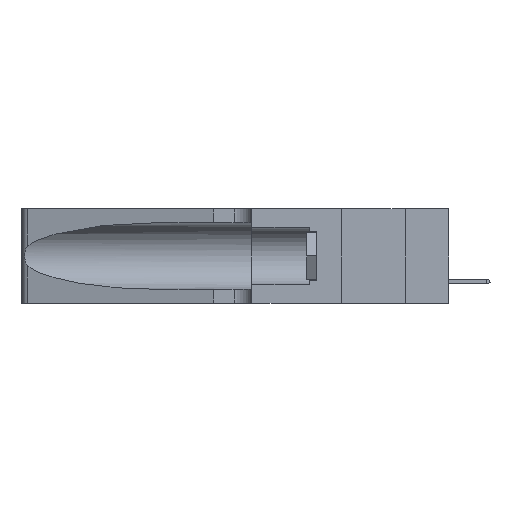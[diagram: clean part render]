
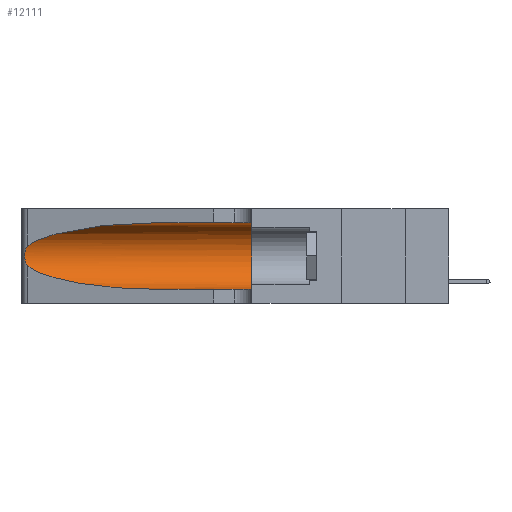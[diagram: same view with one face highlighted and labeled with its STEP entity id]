
A CAD part, left-side view. The second image highlights one B-rep face of the part: STEP entity #12111.
In plain terms, the highlighted cylindrical face has radius 3.308 mm (diameter 6.617 mm), a partial arc.
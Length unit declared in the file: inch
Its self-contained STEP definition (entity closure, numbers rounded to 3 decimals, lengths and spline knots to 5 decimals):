
#416 = CIRCLE ( 'NONE', #11022, 0.13025 ) ;
#434 = CARTESIAN_POINT ( 'NONE',  ( 0.1305, 0.72297, 0.31525 ) ) ;
#457 = DIRECTION ( 'NONE',  ( 0., 0., -1. ) ) ;
#665 = DIRECTION ( 'NONE',  ( 0., -1., 0. ) ) ;
#813 = CARTESIAN_POINT ( 'NONE',  ( 0.1305, 1.61858, 0.05475 ) ) ;
#1003 = EDGE_CURVE ( 'NONE', #6427, #7601, #4981, .T. ) ;
#2131 = CARTESIAN_POINT ( 'NONE',  ( 0.1305, 0.35, 0.185 ) ) ;
#2793 = LINE ( 'NONE', #813, #10927 ) ;
#2992 = EDGE_LOOP ( 'NONE', ( #15662, #5739, #11765, #10380, #9431, #17140 ) ) ;
#3271 = B_SPLINE_CURVE_WITH_KNOTS ( 'NONE', 3,
 ( #14255, #17311, #11623, #3911, #15981, #14503, #13169, #16174, #19158, #14706, #19229, #11430, #14574, #17772 ),
 .UNSPECIFIED., .F., .F.,
 ( 4, 2, 2, 2, 2, 2, 4 ),
 ( 0., 0.00027, 0.00053, 0.00107, 0.0016, 0.00187, 0.00214 ),
 .UNSPECIFIED. ) ;
#3377 = EDGE_CURVE ( 'NONE', #10910, #6811, #11810, .T. ) ;
#3838 = DIRECTION ( 'NONE',  ( 0., -1., 0. ) ) ;
#3911 = CARTESIAN_POINT ( 'NONE',  ( 0.25787, 1.23484, 0.2124 ) ) ;
#4242 = CARTESIAN_POINT ( 'NONE',  ( 0.1305, 1.61858, 0.185 ) ) ;
#4283 = EDGE_CURVE ( 'NONE', #7601, #10910, #3271, .T. ) ;
#4562 = CARTESIAN_POINT ( 'NONE',  ( 0.1305, 0.72297, 0.05475 ) ) ;
#4981 =( BOUNDED_CURVE ( )  B_SPLINE_CURVE ( 3, ( #434, #18572, #14188, #14113 ),
 .UNSPECIFIED., .F., .T. ) 
 B_SPLINE_CURVE_WITH_KNOTS ( ( 4, 4 ),
 ( 1.5708, 2.84003 ),
 .UNSPECIFIED. ) 
 CURVE ( )  GEOMETRIC_REPRESENTATION_ITEM ( )  RATIONAL_B_SPLINE_CURVE ( ( 1., 0.87, 0.87, 1. ) ) 
 REPRESENTATION_ITEM ( '' )  );
#5599 = CARTESIAN_POINT ( 'NONE',  ( 0.1305, 0.35, 0.05475 ) ) ;
#5739 = ORIENTED_EDGE ( 'NONE', *, *, #4283, .T. ) ;
#5906 = VERTEX_POINT ( 'NONE', #5599 ) ;
#6427 = VERTEX_POINT ( 'NONE', #9288 ) ;
#6769 = CYLINDRICAL_SURFACE ( 'NONE', #19738, 0.13025 ) ;
#6794 = EDGE_CURVE ( 'NONE', #6427, #15471, #12425, .T. ) ;
#6811 = VERTEX_POINT ( 'NONE', #19392 ) ;
#7247 = FACE_OUTER_BOUND ( 'NONE', #2992, .T. ) ;
#7505 = CARTESIAN_POINT ( 'NONE',  ( 0.18966, 0.96281, 0.05475 ) ) ;
#7601 = VERTEX_POINT ( 'NONE', #8254 ) ;
#7919 = VECTOR ( 'NONE', #10205, 39.37008 ) ;
#8254 = CARTESIAN_POINT ( 'NONE',  ( 0.25487, 1.22718, 0.22369 ) ) ;
#9288 = CARTESIAN_POINT ( 'NONE',  ( 0.1305, 0.72297, 0.31525 ) ) ;
#9431 = ORIENTED_EDGE ( 'NONE', *, *, #9921, .F. ) ;
#9548 = EDGE_CURVE ( 'NONE', #6811, #5906, #2793, .T. ) ;
#9921 = EDGE_CURVE ( 'NONE', #15471, #5906, #416, .T. ) ;
#10205 = DIRECTION ( 'NONE',  ( 0., -1., 0. ) ) ;
#10380 = ORIENTED_EDGE ( 'NONE', *, *, #9548, .T. ) ;
#10910 = VERTEX_POINT ( 'NONE', #13057 ) ;
#10927 = VECTOR ( 'NONE', #3838, 39.37008 ) ;
#11022 = AXIS2_PLACEMENT_3D ( 'NONE', #2131, #14350, #14552 ) ;
#11430 = CARTESIAN_POINT ( 'NONE',  ( 0.25639, 1.23186, 0.15144 ) ) ;
#11623 = CARTESIAN_POINT ( 'NONE',  ( 0.25639, 1.23184, 0.21858 ) ) ;
#11765 = ORIENTED_EDGE ( 'NONE', *, *, #3377, .T. ) ;
#11810 =( BOUNDED_CURVE ( )  B_SPLINE_CURVE ( 3, ( #15102, #16832, #7505, #4562 ),
 .UNSPECIFIED., .F., .T. ) 
 B_SPLINE_CURVE_WITH_KNOTS ( ( 4, 4 ),
 ( 3.44316, 4.71239 ),
 .UNSPECIFIED. ) 
 CURVE ( )  GEOMETRIC_REPRESENTATION_ITEM ( )  RATIONAL_B_SPLINE_CURVE ( ( 1., 0.87, 0.87, 1. ) ) 
 REPRESENTATION_ITEM ( '' )  );
#12111 = ADVANCED_FACE ( 'NONE', ( #7247 ), #6769, .F. ) ;
#12425 = LINE ( 'NONE', #17932, #7919 ) ;
#13057 = CARTESIAN_POINT ( 'NONE',  ( 0.25487, 1.22718, 0.14631 ) ) ;
#13169 = CARTESIAN_POINT ( 'NONE',  ( 0.26075, 1.23896, 0.19203 ) ) ;
#14113 = CARTESIAN_POINT ( 'NONE',  ( 0.25487, 1.22718, 0.22369 ) ) ;
#14188 = CARTESIAN_POINT ( 'NONE',  ( 0.2373, 1.15595, 0.28018 ) ) ;
#14255 = CARTESIAN_POINT ( 'NONE',  ( 0.25487, 1.22718, 0.22369 ) ) ;
#14350 = DIRECTION ( 'NONE',  ( 0., 1., 0. ) ) ;
#14503 = CARTESIAN_POINT ( 'NONE',  ( 0.26018, 1.23835, 0.19895 ) ) ;
#14552 = DIRECTION ( 'NONE',  ( 0., 0., 1. ) ) ;
#14574 = CARTESIAN_POINT ( 'NONE',  ( 0.25555, 1.22993, 0.14849 ) ) ;
#14706 = CARTESIAN_POINT ( 'NONE',  ( 0.25856, 1.23593, 0.16098 ) ) ;
#15069 = CARTESIAN_POINT ( 'NONE',  ( 0.1305, 0.35, 0.31525 ) ) ;
#15102 = CARTESIAN_POINT ( 'NONE',  ( 0.25487, 1.22718, 0.14631 ) ) ;
#15471 = VERTEX_POINT ( 'NONE', #15069 ) ;
#15662 = ORIENTED_EDGE ( 'NONE', *, *, #1003, .T. ) ;
#15981 = CARTESIAN_POINT ( 'NONE',  ( 0.25854, 1.2359, 0.20912 ) ) ;
#16174 = CARTESIAN_POINT ( 'NONE',  ( 0.26075, 1.23896, 0.178 ) ) ;
#16832 = CARTESIAN_POINT ( 'NONE',  ( 0.2373, 1.15595, 0.08982 ) ) ;
#17140 = ORIENTED_EDGE ( 'NONE', *, *, #6794, .F. ) ;
#17311 = CARTESIAN_POINT ( 'NONE',  ( 0.25555, 1.22994, 0.2215 ) ) ;
#17772 = CARTESIAN_POINT ( 'NONE',  ( 0.25487, 1.22718, 0.14631 ) ) ;
#17932 = CARTESIAN_POINT ( 'NONE',  ( 0.1305, 1.61858, 0.31525 ) ) ;
#18572 = CARTESIAN_POINT ( 'NONE',  ( 0.18966, 0.96281, 0.31525 ) ) ;
#19158 = CARTESIAN_POINT ( 'NONE',  ( 0.26017, 1.23833, 0.17102 ) ) ;
#19229 = CARTESIAN_POINT ( 'NONE',  ( 0.25789, 1.23486, 0.15765 ) ) ;
#19392 = CARTESIAN_POINT ( 'NONE',  ( 0.1305, 0.72297, 0.05475 ) ) ;
#19738 = AXIS2_PLACEMENT_3D ( 'NONE', #4242, #665, #457 ) ;
